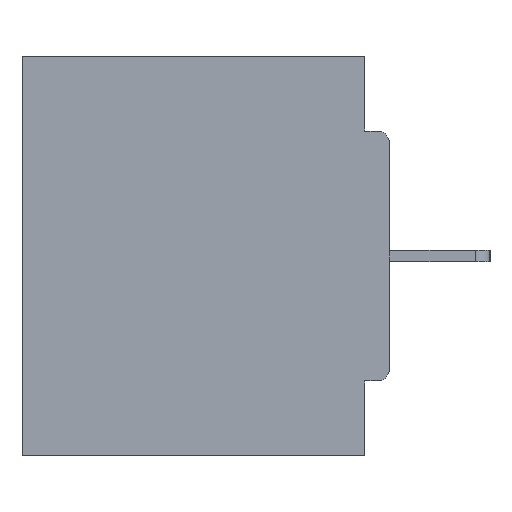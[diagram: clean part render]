
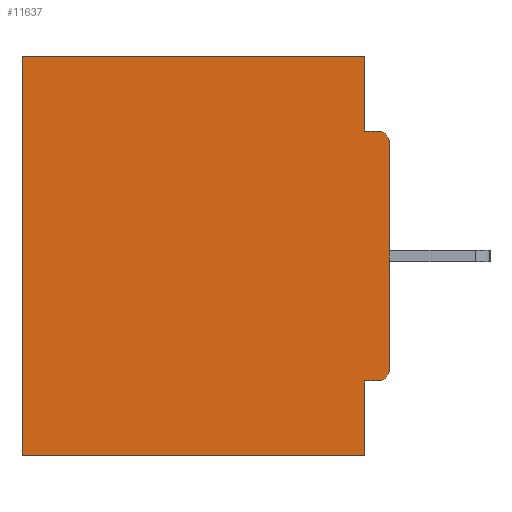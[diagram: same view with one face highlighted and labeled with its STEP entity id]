
A CAD part, left-side view. The second image highlights one B-rep face of the part: STEP entity #11637.
In plain terms, the highlighted planar face has unit normal (-1, 0, 0).
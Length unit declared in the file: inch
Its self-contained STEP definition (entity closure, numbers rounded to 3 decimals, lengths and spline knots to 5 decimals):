
#700 = LINE ( 'NONE', #14981, #11697 ) ;
#888 = ORIENTED_EDGE ( 'NONE', *, *, #4759, .F. ) ;
#1057 = VECTOR ( 'NONE', #14062, 39.37008 ) ;
#1662 = ORIENTED_EDGE ( 'NONE', *, *, #18804, .T. ) ;
#2033 = ORIENTED_EDGE ( 'NONE', *, *, #18375, .F. ) ;
#2471 = ORIENTED_EDGE ( 'NONE', *, *, #19651, .F. ) ;
#2710 = VECTOR ( 'NONE', #7811, 39.37008 ) ;
#3540 = VECTOR ( 'NONE', #15062, 39.37008 ) ;
#3878 = VECTOR ( 'NONE', #7383, 39.37008 ) ;
#3880 = VERTEX_POINT ( 'NONE', #10792 ) ;
#4759 = EDGE_CURVE ( 'NONE', #26314, #5572, #19848, .T. ) ;
#5563 = DIRECTION ( 'NONE',  ( 0., 1., 0. ) ) ;
#5572 = VERTEX_POINT ( 'NONE', #17184 ) ;
#6724 = LINE ( 'NONE', #12795, #11746 ) ;
#7016 = LINE ( 'NONE', #7670, #1057 ) ;
#7160 = VERTEX_POINT ( 'NONE', #22149 ) ;
#7383 = DIRECTION ( 'NONE',  ( 0., 0., -1. ) ) ;
#7670 = CARTESIAN_POINT ( 'NONE',  ( 0.298, 0.031, -0.5 ) ) ;
#7784 = CARTESIAN_POINT ( 'NONE',  ( 0.298, 0., 0. ) ) ;
#7793 = LINE ( 'NONE', #24379, #23913 ) ;
#7811 = DIRECTION ( 'NONE',  ( 0., 1., 0. ) ) ;
#8246 = VERTEX_POINT ( 'NONE', #14246 ) ;
#8538 = DIRECTION ( 'NONE',  ( 0., -1., 0. ) ) ;
#8810 = CARTESIAN_POINT ( 'NONE',  ( 0.298, 0., -0.4065 ) ) ;
#9711 = DIRECTION ( 'NONE',  ( 0., 0., -1. ) ) ;
#10792 = CARTESIAN_POINT ( 'NONE',  ( 0.298, 0.46, 0. ) ) ;
#11159 = CARTESIAN_POINT ( 'NONE',  ( 0.298, 0.015, -0.1085 ) ) ;
#11637 = ADVANCED_FACE ( 'NONE', ( #15698 ), #19018, .F. ) ;
#11697 = VECTOR ( 'NONE', #23354, 39.37008 ) ;
#11746 = VECTOR ( 'NONE', #8538, 39.37008 ) ;
#12139 = CARTESIAN_POINT ( 'NONE',  ( 0.298, 0.031, 0. ) ) ;
#12243 = CARTESIAN_POINT ( 'NONE',  ( 0.298, 0., -0.5 ) ) ;
#12532 = CARTESIAN_POINT ( 'NONE',  ( 0.298, 0.015, -0.3915 ) ) ;
#12726 = DIRECTION ( 'NONE',  ( 0., 0., -1. ) ) ;
#12751 = CIRCLE ( 'NONE', #19071, 0.015 ) ;
#12795 = CARTESIAN_POINT ( 'NONE',  ( 0.298, 0., -0.0935 ) ) ;
#12938 = VERTEX_POINT ( 'NONE', #27487 ) ;
#13260 = DIRECTION ( 'NONE',  ( 0., 0., -1. ) ) ;
#13391 = EDGE_CURVE ( 'NONE', #8246, #14669, #14300, .T. ) ;
#13793 = CARTESIAN_POINT ( 'NONE',  ( 0.298, 0.031, -0.5 ) ) ;
#14062 = DIRECTION ( 'NONE',  ( 0., 0., -1. ) ) ;
#14246 = CARTESIAN_POINT ( 'NONE',  ( 0.298, 0.015, -0.4065 ) ) ;
#14300 = CIRCLE ( 'NONE', #27367, 0.015 ) ;
#14637 = DIRECTION ( 'NONE',  ( 0., 0., -1. ) ) ;
#14669 = VERTEX_POINT ( 'NONE', #15577 ) ;
#14981 = CARTESIAN_POINT ( 'NONE',  ( 0.298, 0.46, 0. ) ) ;
#15062 = DIRECTION ( 'NONE',  ( 0., 1., 0. ) ) ;
#15307 = LINE ( 'NONE', #15797, #3878 ) ;
#15379 = EDGE_CURVE ( 'NONE', #26935, #3880, #25959, .T. ) ;
#15510 = CARTESIAN_POINT ( 'NONE',  ( 0.298, 0., -0.1085 ) ) ;
#15577 = CARTESIAN_POINT ( 'NONE',  ( 0.298, 0., -0.3915 ) ) ;
#15646 = ORIENTED_EDGE ( 'NONE', *, *, #15379, .T. ) ;
#15698 = FACE_OUTER_BOUND ( 'NONE', #16907, .T. ) ;
#15797 = CARTESIAN_POINT ( 'NONE',  ( 0.298, 0., 0. ) ) ;
#16333 = LINE ( 'NONE', #8810, #3540 ) ;
#16763 = ORIENTED_EDGE ( 'NONE', *, *, #26057, .T. ) ;
#16907 = EDGE_LOOP ( 'NONE', ( #1662, #22284, #2471, #15646, #16763, #888, #2033, #23422, #22550, #17265 ) ) ;
#17184 = CARTESIAN_POINT ( 'NONE',  ( 0.298, 0.46, -0.5 ) ) ;
#17265 = ORIENTED_EDGE ( 'NONE', *, *, #19574, .F. ) ;
#18375 = EDGE_CURVE ( 'NONE', #7160, #26314, #7793, .T. ) ;
#18645 = VERTEX_POINT ( 'NONE', #21125 ) ;
#18804 = EDGE_CURVE ( 'NONE', #24148, #12938, #12751, .T. ) ;
#19018 = PLANE ( 'NONE',  #26324 ) ;
#19071 = AXIS2_PLACEMENT_3D ( 'NONE', #11159, #25769, #13260 ) ;
#19361 = EDGE_CURVE ( 'NONE', #8246, #7160, #16333, .T. ) ;
#19574 = EDGE_CURVE ( 'NONE', #24148, #14669, #15307, .T. ) ;
#19651 = EDGE_CURVE ( 'NONE', #26935, #18645, #7016, .T. ) ;
#19848 = LINE ( 'NONE', #12243, #2710 ) ;
#20502 = VECTOR ( 'NONE', #5563, 39.37008 ) ;
#21115 = CARTESIAN_POINT ( 'NONE',  ( 0.298, 0., 0. ) ) ;
#21125 = CARTESIAN_POINT ( 'NONE',  ( 0.298, 0.031, -0.0935 ) ) ;
#22149 = CARTESIAN_POINT ( 'NONE',  ( 0.298, 0.031, -0.4065 ) ) ;
#22284 = ORIENTED_EDGE ( 'NONE', *, *, #25199, .F. ) ;
#22550 = ORIENTED_EDGE ( 'NONE', *, *, #13391, .T. ) ;
#23354 = DIRECTION ( 'NONE',  ( 0., 0., -1. ) ) ;
#23422 = ORIENTED_EDGE ( 'NONE', *, *, #19361, .F. ) ;
#23913 = VECTOR ( 'NONE', #9711, 39.37008 ) ;
#24148 = VERTEX_POINT ( 'NONE', #15510 ) ;
#24379 = CARTESIAN_POINT ( 'NONE',  ( 0.298, 0.031, -0.5 ) ) ;
#25199 = EDGE_CURVE ( 'NONE', #18645, #12938, #6724, .T. ) ;
#25246 = DIRECTION ( 'NONE',  ( 1., 0., 0. ) ) ;
#25769 = DIRECTION ( 'NONE',  ( -1., 0., 0. ) ) ;
#25959 = LINE ( 'NONE', #7784, #20502 ) ;
#26057 = EDGE_CURVE ( 'NONE', #3880, #5572, #700, .T. ) ;
#26314 = VERTEX_POINT ( 'NONE', #13793 ) ;
#26324 = AXIS2_PLACEMENT_3D ( 'NONE', #21115, #25246, #12726 ) ;
#26935 = VERTEX_POINT ( 'NONE', #12139 ) ;
#27121 = DIRECTION ( 'NONE',  ( -1., 0., 0. ) ) ;
#27367 = AXIS2_PLACEMENT_3D ( 'NONE', #12532, #27121, #14637 ) ;
#27487 = CARTESIAN_POINT ( 'NONE',  ( 0.298, 0.015, -0.0935 ) ) ;
